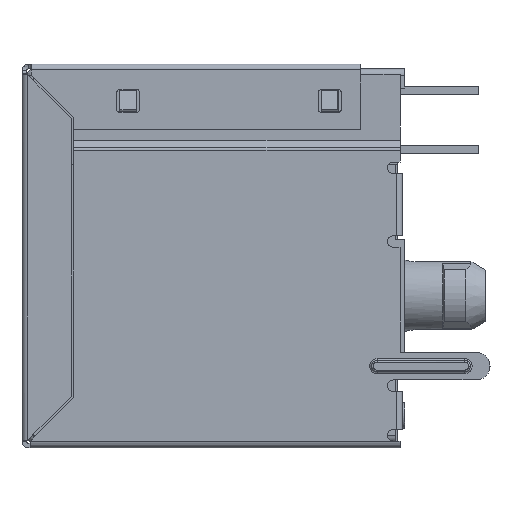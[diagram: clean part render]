
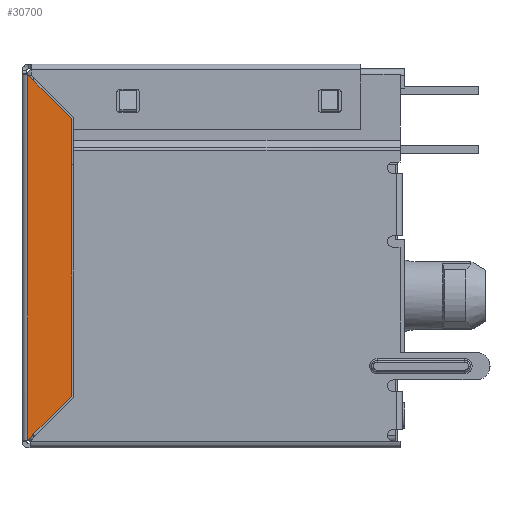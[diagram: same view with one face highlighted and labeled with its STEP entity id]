
A CAD part, left-side view. The second image highlights one B-rep face of the part: STEP entity #30700.
In plain terms, the highlighted planar face has unit normal (-1, 0, 0).
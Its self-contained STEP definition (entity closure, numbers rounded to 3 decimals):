
#1003 = VECTOR ( 'NONE', #37339, 1000. ) ;
#2566 = FACE_OUTER_BOUND ( 'NONE', #8185, .T. ) ;
#2575 = CARTESIAN_POINT ( 'NONE',  ( -7.95, -0.05, -6.303 ) ) ;
#3149 = EDGE_CURVE ( 'NONE', #20079, #30228, #15713, .T. ) ;
#4040 = EDGE_CURVE ( 'NONE', #20079, #7698, #28958, .T. ) ;
#5611 = VECTOR ( 'NONE', #13411, 1000. ) ;
#6951 = VECTOR ( 'NONE', #32931, 1000. ) ;
#7244 = ORIENTED_EDGE ( 'NONE', *, *, #27303, .T. ) ;
#7698 = VERTEX_POINT ( 'NONE', #19211 ) ;
#8185 = EDGE_LOOP ( 'NONE', ( #9383, #7244, #13382, #16396 ) ) ;
#8418 = AXIS2_PLACEMENT_3D ( 'NONE', #34781, #11600, #28910 ) ;
#9383 = ORIENTED_EDGE ( 'NONE', *, *, #3149, .T. ) ;
#11600 = DIRECTION ( 'NONE',  ( 1., 0., 0. ) ) ;
#13382 = ORIENTED_EDGE ( 'NONE', *, *, #27349, .T. ) ;
#13411 = DIRECTION ( 'NONE',  ( 0., 0., 1. ) ) ;
#15713 = LINE ( 'NONE', #19123, #6951 ) ;
#16396 = ORIENTED_EDGE ( 'NONE', *, *, #4040, .F. ) ;
#19123 = CARTESIAN_POINT ( 'NONE',  ( -7.95, -0.009, -6.303 ) ) ;
#19211 = CARTESIAN_POINT ( 'NONE',  ( -7.95, -0.05, 9.582 ) ) ;
#20079 = VERTEX_POINT ( 'NONE', #23507 ) ;
#21054 = CARTESIAN_POINT ( 'NONE',  ( -7.95, -1.95, 7.682 ) ) ;
#21188 = VECTOR ( 'NONE', #25970, 1000. ) ;
#21416 = CARTESIAN_POINT ( 'NONE',  ( -7.95, -1.95, -4.361 ) ) ;
#22525 = VERTEX_POINT ( 'NONE', #21054 ) ;
#23054 = PLANE ( 'NONE',  #8418 ) ;
#23507 = CARTESIAN_POINT ( 'NONE',  ( -7.95, -0.05, -6.261 ) ) ;
#25858 = CARTESIAN_POINT ( 'NONE',  ( -7.95, 0., 9.632 ) ) ;
#25970 = DIRECTION ( 'NONE',  ( 0., 0., 1. ) ) ;
#27303 = EDGE_CURVE ( 'NONE', #30228, #22525, #37247, .T. ) ;
#27349 = EDGE_CURVE ( 'NONE', #22525, #7698, #29483, .T. ) ;
#28910 = DIRECTION ( 'NONE',  ( 0., 1., 0. ) ) ;
#28958 = LINE ( 'NONE', #2575, #21188 ) ;
#29483 = LINE ( 'NONE', #25858, #1003 ) ;
#30228 = VERTEX_POINT ( 'NONE', #21416 ) ;
#30700 = ADVANCED_FACE ( 'NONE', ( #2566 ), #23054, .F. ) ;
#32931 = DIRECTION ( 'NONE',  ( 0., -0.707, 0.707 ) ) ;
#33781 = CARTESIAN_POINT ( 'NONE',  ( -7.95, -1.95, 7.682 ) ) ;
#34781 = CARTESIAN_POINT ( 'NONE',  ( -7.95, 0., -6.303 ) ) ;
#37247 = LINE ( 'NONE', #33781, #5611 ) ;
#37339 = DIRECTION ( 'NONE',  ( 0., 0.707, 0.707 ) ) ;
